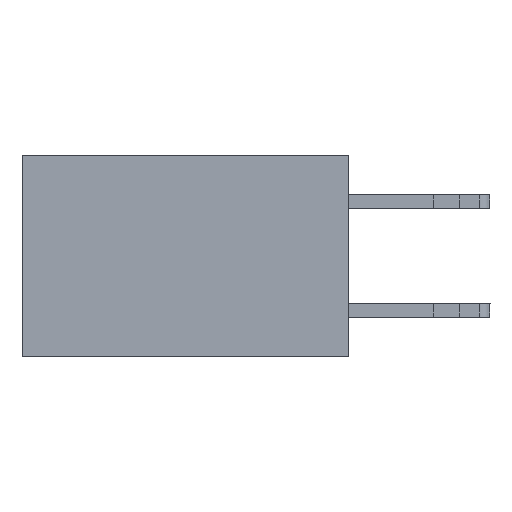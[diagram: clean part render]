
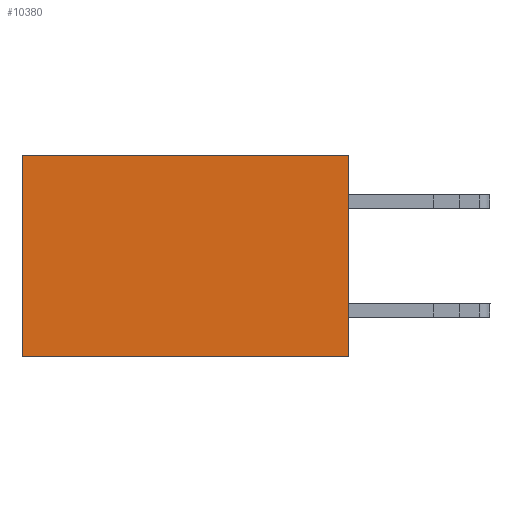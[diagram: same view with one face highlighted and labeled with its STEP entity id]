
A CAD part, left-side view. The second image highlights one B-rep face of the part: STEP entity #10380.
In plain terms, the highlighted planar face has unit normal (-1, 0, 0).
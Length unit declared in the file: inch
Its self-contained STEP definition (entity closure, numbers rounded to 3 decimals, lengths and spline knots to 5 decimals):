
#69 = ORIENTED_EDGE ( 'NONE', *, *, #15014, .T. ) ;
#748 = DIRECTION ( 'NONE',  ( 0., 0., -1. ) ) ;
#1411 = DIRECTION ( 'NONE',  ( 0., 0., -1. ) ) ;
#1495 = EDGE_LOOP ( 'NONE', ( #69, #1835, #11670, #10964 ) ) ;
#1835 = ORIENTED_EDGE ( 'NONE', *, *, #3499, .F. ) ;
#3336 = EDGE_CURVE ( 'NONE', #6077, #3972, #9672, .T. ) ;
#3499 = EDGE_CURVE ( 'NONE', #3972, #15270, #6836, .T. ) ;
#3972 = VERTEX_POINT ( 'NONE', #4113 ) ;
#4113 = CARTESIAN_POINT ( 'NONE',  ( 0.2615, 0., -0.37 ) ) ;
#4812 = VECTOR ( 'NONE', #17089, 39.37008 ) ;
#5737 = CARTESIAN_POINT ( 'NONE',  ( 0.2615, 0.6, -0.37 ) ) ;
#5789 = PLANE ( 'NONE',  #10594 ) ;
#6077 = VERTEX_POINT ( 'NONE', #17254 ) ;
#6836 = LINE ( 'NONE', #8140, #7026 ) ;
#7026 = VECTOR ( 'NONE', #7799, 39.37008 ) ;
#7266 = CARTESIAN_POINT ( 'NONE',  ( 0.2615, 0., 0. ) ) ;
#7579 = CARTESIAN_POINT ( 'NONE',  ( 0.2615, 0.6, 0. ) ) ;
#7799 = DIRECTION ( 'NONE',  ( 0., 1., 0. ) ) ;
#8008 = CARTESIAN_POINT ( 'NONE',  ( 0.2615, 0.6, -0.37 ) ) ;
#8140 = CARTESIAN_POINT ( 'NONE',  ( 0.2615, 0., -0.37 ) ) ;
#8598 = LINE ( 'NONE', #8008, #16101 ) ;
#8707 = FACE_OUTER_BOUND ( 'NONE', #1495, .T. ) ;
#9446 = LINE ( 'NONE', #7266, #4812 ) ;
#9672 = LINE ( 'NONE', #10634, #16714 ) ;
#10045 = DIRECTION ( 'NONE',  ( 1., 0., 0. ) ) ;
#10380 = ADVANCED_FACE ( 'NONE', ( #8707 ), #5789, .F. ) ;
#10594 = AXIS2_PLACEMENT_3D ( 'NONE', #18394, #10045, #1411 ) ;
#10634 = CARTESIAN_POINT ( 'NONE',  ( 0.2615, 0., -0.37 ) ) ;
#10647 = DIRECTION ( 'NONE',  ( 0., 0., -1. ) ) ;
#10964 = ORIENTED_EDGE ( 'NONE', *, *, #16335, .T. ) ;
#11670 = ORIENTED_EDGE ( 'NONE', *, *, #3336, .F. ) ;
#11885 = VERTEX_POINT ( 'NONE', #7579 ) ;
#15014 = EDGE_CURVE ( 'NONE', #11885, #15270, #8598, .T. ) ;
#15270 = VERTEX_POINT ( 'NONE', #5737 ) ;
#16101 = VECTOR ( 'NONE', #748, 39.37008 ) ;
#16335 = EDGE_CURVE ( 'NONE', #6077, #11885, #9446, .T. ) ;
#16714 = VECTOR ( 'NONE', #10647, 39.37008 ) ;
#17089 = DIRECTION ( 'NONE',  ( 0., 1., 0. ) ) ;
#17254 = CARTESIAN_POINT ( 'NONE',  ( 0.2615, 0., 0. ) ) ;
#18394 = CARTESIAN_POINT ( 'NONE',  ( 0.2615, 0., -0.37 ) ) ;
